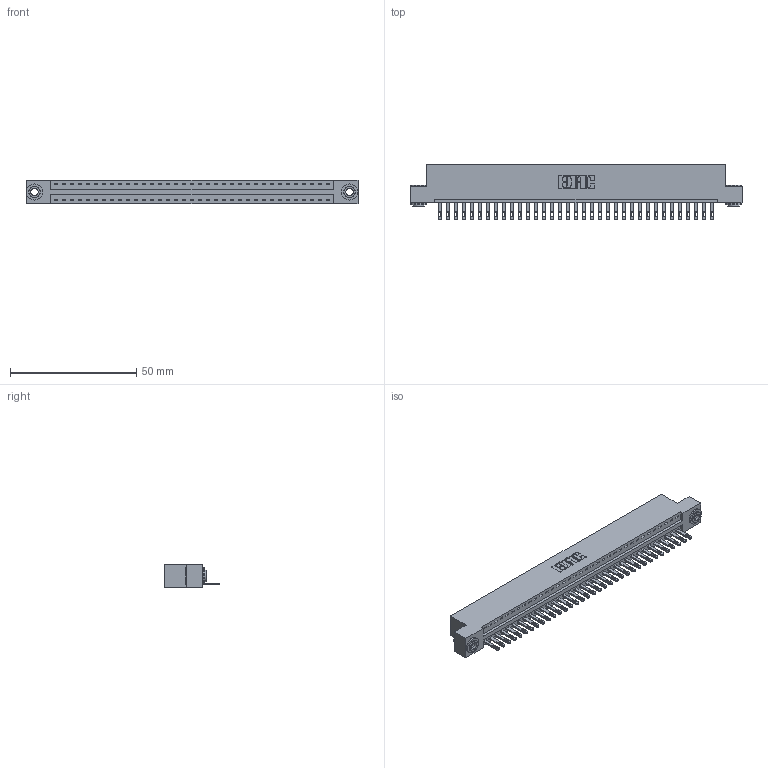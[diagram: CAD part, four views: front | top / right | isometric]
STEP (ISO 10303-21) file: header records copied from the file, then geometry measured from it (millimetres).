
FILE_DESCRIPTION (( 'STEP AP203' ), '1' );
FILE_NAME ('896-035-500-103.STEP', '2021-07-27T19:55:45', ( '' ), ( '' ), 'SwSTEP 2.0', 'SolidWorks 2020', '' );
FILE_SCHEMA (( 'CONFIG_CONTROL_DESIGN' ));
Length unit declared in the file: inch
Products named in the file (4): 345-250-002_345-250-002-102; 846 Part_Flush Mounting Lugs - 0.156 Dia-TH; 345-292-001_345-293-100; 896-035-500-103
Assembly tree (38 placements, depth 2):
  896-035-500-103
    846 Part_Flush Mounting Lugs - 0.156 Dia-TH
    345-292-001_345-293-100  x35
    345-250-002_345-250-002-102  x2
Bounding box: 131.7 x 21.84 x 9.4 mm (x, y, z)
Volume: 12599.3 mm3; surface area: 15972.7 mm2
Topology: 38 solids, 38 shells, 2050 faces, 6285 edges, 4186 vertices
Faces by surface type: plane 1276, cylinder 766, cone 8
Entity records: 23244 total; most frequent: CARTESIAN_POINT 3964, ORIENTED_EDGE 3926, DIRECTION 3539, EDGE_CURVE 1963, VECTOR 1663, LINE 1663, VERTEX_POINT 1306, AXIS2_PLACEMENT_3D 938
